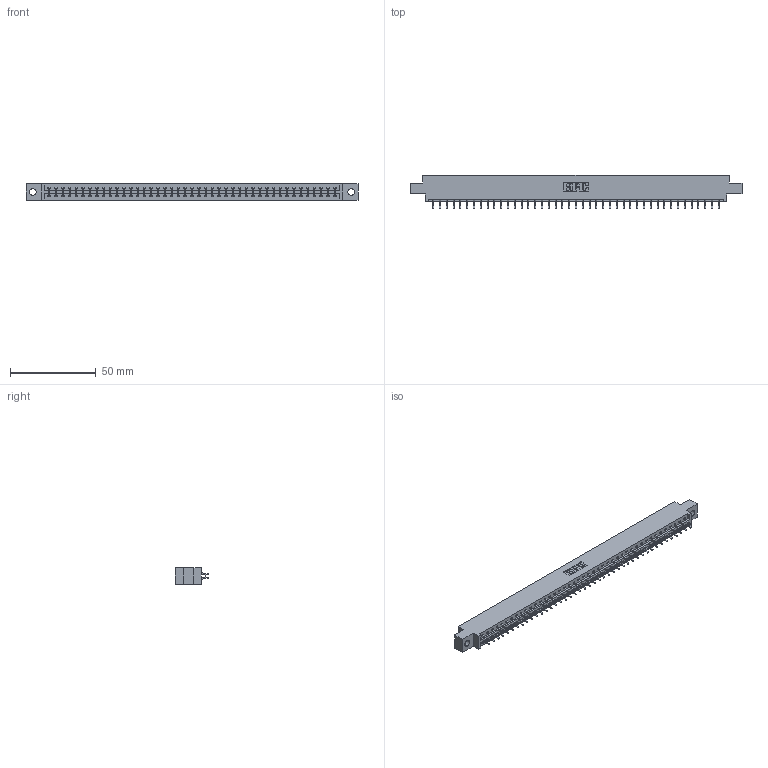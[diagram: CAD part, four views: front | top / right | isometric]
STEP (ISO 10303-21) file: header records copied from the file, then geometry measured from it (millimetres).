
FILE_DESCRIPTION (( 'STEP AP203' ), '1' );
FILE_NAME ('387-086-556-804.STEP', '2019-10-23T04:19:31', ( '' ), ( '' ), 'SwSTEP 2.0', 'SolidWorks 2016', '' );
FILE_SCHEMA (( 'CONFIG_CONTROL_DESIGN' ));
Length unit declared in the file: inch
Products named in the file (3): 337 Part_0.170 Offset - 0.156 Dia-TH; 387-086-556-804; 345-292-001_556 Tail
Assembly tree (87 placements, depth 2):
  387-086-556-804
    337 Part_0.170 Offset - 0.156 Dia-TH
    345-292-001_556 Tail  x86
Bounding box: 193.4 x 19.57 x 9.4 mm (x, y, z)
Volume: 20186.1 mm3; surface area: 22644.6 mm2
Topology: 87 solids, 87 shells, 5278 faces, 15717 edges, 10362 vertices
Faces by surface type: plane 3686, cylinder 1592
Entity records: 33565 total; most frequent: CARTESIAN_POINT 5670, ORIENTED_EDGE 5594, DIRECTION 4809, EDGE_CURVE 2797, VECTOR 2661, LINE 2661, VERTEX_POINT 1862, AXIS2_PLACEMENT_3D 1074
